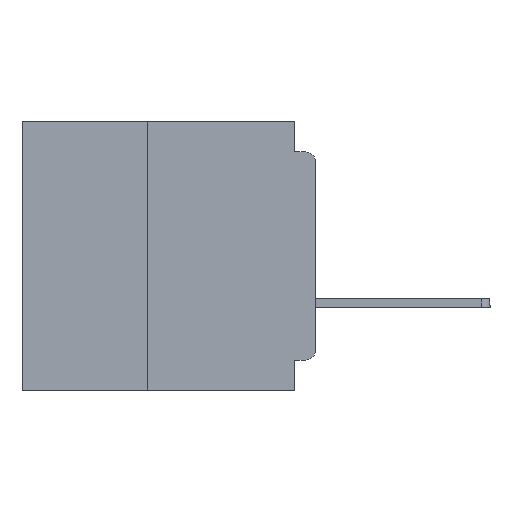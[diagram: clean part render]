
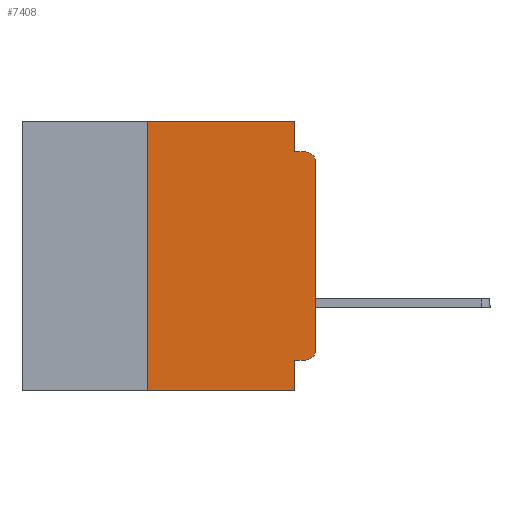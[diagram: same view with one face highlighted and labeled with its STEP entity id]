
A CAD part, left-side view. The second image highlights one B-rep face of the part: STEP entity #7408.
In plain terms, the highlighted planar face has unit normal (-1, 0, 0).
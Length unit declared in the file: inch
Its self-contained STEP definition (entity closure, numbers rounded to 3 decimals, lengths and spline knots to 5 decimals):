
#860 = LINE ( 'NONE', #34823, #7797 ) ;
#1919 = CARTESIAN_POINT ( 'NONE',  ( 0., 0.015, -0.06 ) ) ;
#2370 = LINE ( 'NONE', #31581, #23590 ) ;
#2397 = VECTOR ( 'NONE', #24348, 39.37008 ) ;
#3050 = VERTEX_POINT ( 'NONE', #27109 ) ;
#3189 = LINE ( 'NONE', #19295, #17704 ) ;
#3361 = CARTESIAN_POINT ( 'NONE',  ( 0., 0.015, -0.355 ) ) ;
#4229 = CARTESIAN_POINT ( 'NONE',  ( 0., 0.031, 0. ) ) ;
#4472 = DIRECTION ( 'NONE',  ( 0., 0., -1. ) ) ;
#4652 = EDGE_CURVE ( 'NONE', #21919, #17782, #25093, .T. ) ;
#4914 = DIRECTION ( 'NONE',  ( 0., 0., -1. ) ) ;
#4922 = DIRECTION ( 'NONE',  ( 0., -1., 0. ) ) ;
#4971 = ORIENTED_EDGE ( 'NONE', *, *, #25317, .F. ) ;
#6505 = VERTEX_POINT ( 'NONE', #25990 ) ;
#6926 = ORIENTED_EDGE ( 'NONE', *, *, #15363, .F. ) ;
#7163 = VERTEX_POINT ( 'NONE', #28863 ) ;
#7408 = ADVANCED_FACE ( 'NONE', ( #21935 ), #13141, .F. ) ;
#7479 = EDGE_LOOP ( 'NONE', ( #24953, #14768, #24609, #23541, #6926, #19636, #17111, #23388, #4971, #15920 ) ) ;
#7652 = CARTESIAN_POINT ( 'NONE',  ( 0., 0.031, -0.045 ) ) ;
#7797 = VECTOR ( 'NONE', #26443, 39.37008 ) ;
#10440 = DIRECTION ( 'NONE',  ( -1., 0., 0. ) ) ;
#10893 = LINE ( 'NONE', #27225, #16692 ) ;
#12041 = CARTESIAN_POINT ( 'NONE',  ( 0., 0.031, -0.355 ) ) ;
#12958 = VERTEX_POINT ( 'NONE', #3361 ) ;
#13141 = PLANE ( 'NONE',  #23180 ) ;
#13302 = VERTEX_POINT ( 'NONE', #16657 ) ;
#13533 = AXIS2_PLACEMENT_3D ( 'NONE', #27432, #10440, #30271 ) ;
#13650 = CARTESIAN_POINT ( 'NONE',  ( 0., 0.015, -0.045 ) ) ;
#14768 = ORIENTED_EDGE ( 'NONE', *, *, #33782, .T. ) ;
#15363 = EDGE_CURVE ( 'NONE', #7163, #3050, #32890, .T. ) ;
#15920 = ORIENTED_EDGE ( 'NONE', *, *, #31988, .T. ) ;
#16058 = LINE ( 'NONE', #4229, #2397 ) ;
#16657 = CARTESIAN_POINT ( 'NONE',  ( 0., 0., -0.06 ) ) ;
#16692 = VECTOR ( 'NONE', #30065, 39.37008 ) ;
#17111 = ORIENTED_EDGE ( 'NONE', *, *, #24979, .T. ) ;
#17288 = AXIS2_PLACEMENT_3D ( 'NONE', #1919, #22164, #4914 ) ;
#17704 = VECTOR ( 'NONE', #4922, 39.37008 ) ;
#17782 = VERTEX_POINT ( 'NONE', #13650 ) ;
#19295 = CARTESIAN_POINT ( 'NONE',  ( 0., 0.437, -0.4 ) ) ;
#19636 = ORIENTED_EDGE ( 'NONE', *, *, #36213, .F. ) ;
#19696 = VERTEX_POINT ( 'NONE', #25427 ) ;
#19840 = EDGE_CURVE ( 'NONE', #32332, #34144, #2370, .T. ) ;
#20366 = DIRECTION ( 'NONE',  ( 0., 0., -1. ) ) ;
#21103 = CIRCLE ( 'NONE', #13533, 0.015 ) ;
#21758 = DIRECTION ( 'NONE',  ( 1., 0., 0. ) ) ;
#21919 = VERTEX_POINT ( 'NONE', #7652 ) ;
#21935 = FACE_OUTER_BOUND ( 'NONE', #7479, .T. ) ;
#22164 = DIRECTION ( 'NONE',  ( -1., 0., 0. ) ) ;
#23180 = AXIS2_PLACEMENT_3D ( 'NONE', #35631, #21758, #4472 ) ;
#23388 = ORIENTED_EDGE ( 'NONE', *, *, #19840, .F. ) ;
#23541 = ORIENTED_EDGE ( 'NONE', *, *, #28629, .F. ) ;
#23590 = VECTOR ( 'NONE', #20366, 39.37008 ) ;
#24348 = DIRECTION ( 'NONE',  ( 0., 0., -1. ) ) ;
#24609 = ORIENTED_EDGE ( 'NONE', *, *, #4652, .F. ) ;
#24953 = ORIENTED_EDGE ( 'NONE', *, *, #31257, .T. ) ;
#24979 = EDGE_CURVE ( 'NONE', #19696, #34144, #3189, .T. ) ;
#25093 = LINE ( 'NONE', #29873, #31703 ) ;
#25317 = EDGE_CURVE ( 'NONE', #12958, #32332, #860, .T. ) ;
#25427 = CARTESIAN_POINT ( 'NONE',  ( 0., 0.25, -0.4 ) ) ;
#25990 = CARTESIAN_POINT ( 'NONE',  ( 0., 0., -0.34 ) ) ;
#26443 = DIRECTION ( 'NONE',  ( 0., 1., 0. ) ) ;
#27109 = CARTESIAN_POINT ( 'NONE',  ( 0., 0.031, 0. ) ) ;
#27225 = CARTESIAN_POINT ( 'NONE',  ( 0., 0., 0. ) ) ;
#27432 = CARTESIAN_POINT ( 'NONE',  ( 0., 0.015, -0.34 ) ) ;
#27843 = CARTESIAN_POINT ( 'NONE',  ( 0., 0.25, -0.4 ) ) ;
#28053 = CARTESIAN_POINT ( 'NONE',  ( 0., 0.437, 0. ) ) ;
#28629 = EDGE_CURVE ( 'NONE', #3050, #21919, #16058, .T. ) ;
#28863 = CARTESIAN_POINT ( 'NONE',  ( 0., 0.25, 0. ) ) ;
#29786 = DIRECTION ( 'NONE',  ( 0., -1., 0. ) ) ;
#29873 = CARTESIAN_POINT ( 'NONE',  ( 0., 0., -0.045 ) ) ;
#29942 = VECTOR ( 'NONE', #30693, 39.37008 ) ;
#30065 = DIRECTION ( 'NONE',  ( 0., 0., 1. ) ) ;
#30271 = DIRECTION ( 'NONE',  ( 0., 0., -1. ) ) ;
#30693 = DIRECTION ( 'NONE',  ( 0., 0., 1. ) ) ;
#31118 = VECTOR ( 'NONE', #33741, 39.37008 ) ;
#31257 = EDGE_CURVE ( 'NONE', #6505, #13302, #10893, .T. ) ;
#31521 = CIRCLE ( 'NONE', #17288, 0.015 ) ;
#31581 = CARTESIAN_POINT ( 'NONE',  ( 0., 0.031, -0.4 ) ) ;
#31703 = VECTOR ( 'NONE', #29786, 39.37008 ) ;
#31723 = LINE ( 'NONE', #27843, #29942 ) ;
#31988 = EDGE_CURVE ( 'NONE', #12958, #6505, #21103, .T. ) ;
#32103 = CARTESIAN_POINT ( 'NONE',  ( 0., 0.031, -0.4 ) ) ;
#32332 = VERTEX_POINT ( 'NONE', #12041 ) ;
#32890 = LINE ( 'NONE', #28053, #31118 ) ;
#33741 = DIRECTION ( 'NONE',  ( 0., -1., 0. ) ) ;
#33782 = EDGE_CURVE ( 'NONE', #13302, #17782, #31521, .T. ) ;
#34144 = VERTEX_POINT ( 'NONE', #32103 ) ;
#34823 = CARTESIAN_POINT ( 'NONE',  ( 0., 0., -0.355 ) ) ;
#35631 = CARTESIAN_POINT ( 'NONE',  ( 0., 0.437, 0. ) ) ;
#36213 = EDGE_CURVE ( 'NONE', #19696, #7163, #31723, .T. ) ;
